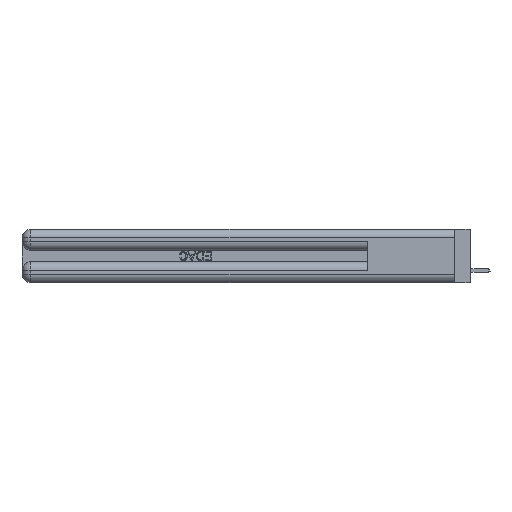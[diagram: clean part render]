
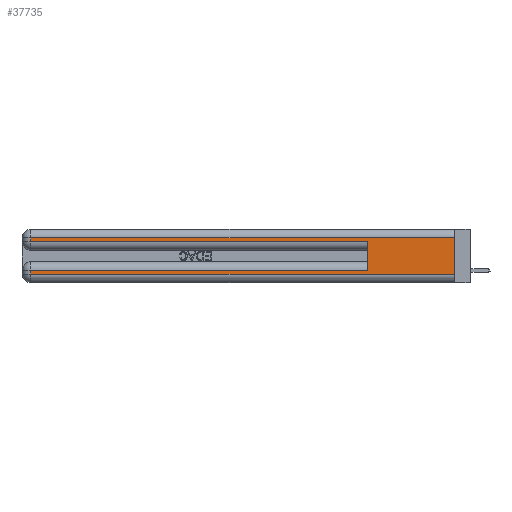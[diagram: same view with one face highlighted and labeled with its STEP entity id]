
A CAD part, left-side view. The second image highlights one B-rep face of the part: STEP entity #37735.
In plain terms, the highlighted planar face has unit normal (-1, 0, 0).
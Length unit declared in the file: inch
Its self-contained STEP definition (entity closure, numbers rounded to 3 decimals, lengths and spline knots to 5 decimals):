
#97 = LINE ( 'NONE', #15990, #8535 ) ;
#202 = ORIENTED_EDGE ( 'NONE', *, *, #12167, .T. ) ;
#1380 = DIRECTION ( 'NONE',  ( 0., 1., 0. ) ) ;
#1959 = DIRECTION ( 'NONE',  ( 0., 0., -1. ) ) ;
#2107 = DIRECTION ( 'NONE',  ( 0., 0., -1. ) ) ;
#2696 = LINE ( 'NONE', #23165, #15035 ) ;
#2721 = DIRECTION ( 'NONE',  ( 1., 0., 0. ) ) ;
#2989 = CARTESIAN_POINT ( 'NONE',  ( 0., 0., 0.285 ) ) ;
#3702 = VECTOR ( 'NONE', #2107, 39.37008 ) ;
#4845 = CARTESIAN_POINT ( 'NONE',  ( 0., 0., 0.06 ) ) ;
#6970 = PLANE ( 'NONE',  #7227 ) ;
#7227 = AXIS2_PLACEMENT_3D ( 'NONE', #35668, #2721, #10174 ) ;
#8423 = DIRECTION ( 'NONE',  ( 0., 0., -1. ) ) ;
#8535 = VECTOR ( 'NONE', #1959, 39.37008 ) ;
#8787 = LINE ( 'NONE', #30877, #3702 ) ;
#10174 = DIRECTION ( 'NONE',  ( 0., 0., -1. ) ) ;
#11442 = LINE ( 'NONE', #22789, #36922 ) ;
#11812 = DIRECTION ( 'NONE',  ( 0., -1., 0. ) ) ;
#12167 = EDGE_CURVE ( 'NONE', #35138, #42969, #42389, .T. ) ;
#12433 = CARTESIAN_POINT ( 'NONE',  ( 0., 0.6, 0.285 ) ) ;
#12618 = ORIENTED_EDGE ( 'NONE', *, *, #20553, .F. ) ;
#15035 = VECTOR ( 'NONE', #28261, 39.37008 ) ;
#15878 = EDGE_CURVE ( 'NONE', #24091, #18777, #42020, .T. ) ;
#15990 = CARTESIAN_POINT ( 'NONE',  ( 0., 2.94, 0.37 ) ) ;
#16356 = CARTESIAN_POINT ( 'NONE',  ( 0., 0., 0.06 ) ) ;
#18661 = FACE_OUTER_BOUND ( 'NONE', #31750, .T. ) ;
#18777 = VERTEX_POINT ( 'NONE', #12433 ) ;
#20553 = EDGE_CURVE ( 'NONE', #22888, #18777, #2696, .T. ) ;
#21402 = CARTESIAN_POINT ( 'NONE',  ( 0., 0., 0.31 ) ) ;
#21590 = EDGE_CURVE ( 'NONE', #30328, #35138, #8787, .T. ) ;
#21641 = LINE ( 'NONE', #21402, #30097 ) ;
#22131 = DIRECTION ( 'NONE',  ( 0., 1., 0. ) ) ;
#22789 = CARTESIAN_POINT ( 'NONE',  ( 0., 0., 0.37 ) ) ;
#22888 = VERTEX_POINT ( 'NONE', #32637 ) ;
#23165 = CARTESIAN_POINT ( 'NONE',  ( 0., 0.6, 0.145 ) ) ;
#24091 = VERTEX_POINT ( 'NONE', #45761 ) ;
#24571 = EDGE_CURVE ( 'NONE', #27538, #24091, #97, .T. ) ;
#25040 = EDGE_CURVE ( 'NONE', #27846, #27538, #21641, .T. ) ;
#26347 = CARTESIAN_POINT ( 'NONE',  ( 0., 0., 0.085 ) ) ;
#27538 = VERTEX_POINT ( 'NONE', #40131 ) ;
#27846 = VERTEX_POINT ( 'NONE', #37782 ) ;
#28246 = VECTOR ( 'NONE', #11812, 39.37008 ) ;
#28261 = DIRECTION ( 'NONE',  ( 0., 0., 1. ) ) ;
#28787 = ORIENTED_EDGE ( 'NONE', *, *, #24571, .T. ) ;
#30069 = VECTOR ( 'NONE', #42865, 39.37008 ) ;
#30097 = VECTOR ( 'NONE', #22131, 39.37008 ) ;
#30328 = VERTEX_POINT ( 'NONE', #38702 ) ;
#30613 = EDGE_CURVE ( 'NONE', #22888, #30328, #34811, .T. ) ;
#30877 = CARTESIAN_POINT ( 'NONE',  ( 0., 2.94, 0.37 ) ) ;
#30901 = CARTESIAN_POINT ( 'NONE',  ( 0., 2.94, 0.06 ) ) ;
#31750 = EDGE_LOOP ( 'NONE', ( #45690, #32798, #28787, #31770, #12618, #41921, #39279, #202 ) ) ;
#31770 = ORIENTED_EDGE ( 'NONE', *, *, #15878, .T. ) ;
#32637 = CARTESIAN_POINT ( 'NONE',  ( 0., 0.6, 0.085 ) ) ;
#32798 = ORIENTED_EDGE ( 'NONE', *, *, #25040, .T. ) ;
#34811 = LINE ( 'NONE', #26347, #39305 ) ;
#35138 = VERTEX_POINT ( 'NONE', #30901 ) ;
#35668 = CARTESIAN_POINT ( 'NONE',  ( 0., 0., 0.37 ) ) ;
#36922 = VECTOR ( 'NONE', #8423, 39.37008 ) ;
#37735 = ADVANCED_FACE ( 'NONE', ( #18661 ), #6970, .F. ) ;
#37782 = CARTESIAN_POINT ( 'NONE',  ( 0., 0., 0.31 ) ) ;
#38702 = CARTESIAN_POINT ( 'NONE',  ( 0., 2.94, 0.085 ) ) ;
#39279 = ORIENTED_EDGE ( 'NONE', *, *, #21590, .T. ) ;
#39305 = VECTOR ( 'NONE', #1380, 39.37008 ) ;
#40131 = CARTESIAN_POINT ( 'NONE',  ( 0., 2.94, 0.31 ) ) ;
#41921 = ORIENTED_EDGE ( 'NONE', *, *, #30613, .T. ) ;
#42020 = LINE ( 'NONE', #2989, #30069 ) ;
#42389 = LINE ( 'NONE', #4845, #28246 ) ;
#42865 = DIRECTION ( 'NONE',  ( 0., -1., 0. ) ) ;
#42969 = VERTEX_POINT ( 'NONE', #16356 ) ;
#44362 = EDGE_CURVE ( 'NONE', #27846, #42969, #11442, .T. ) ;
#45690 = ORIENTED_EDGE ( 'NONE', *, *, #44362, .F. ) ;
#45761 = CARTESIAN_POINT ( 'NONE',  ( 0., 2.94, 0.285 ) ) ;
